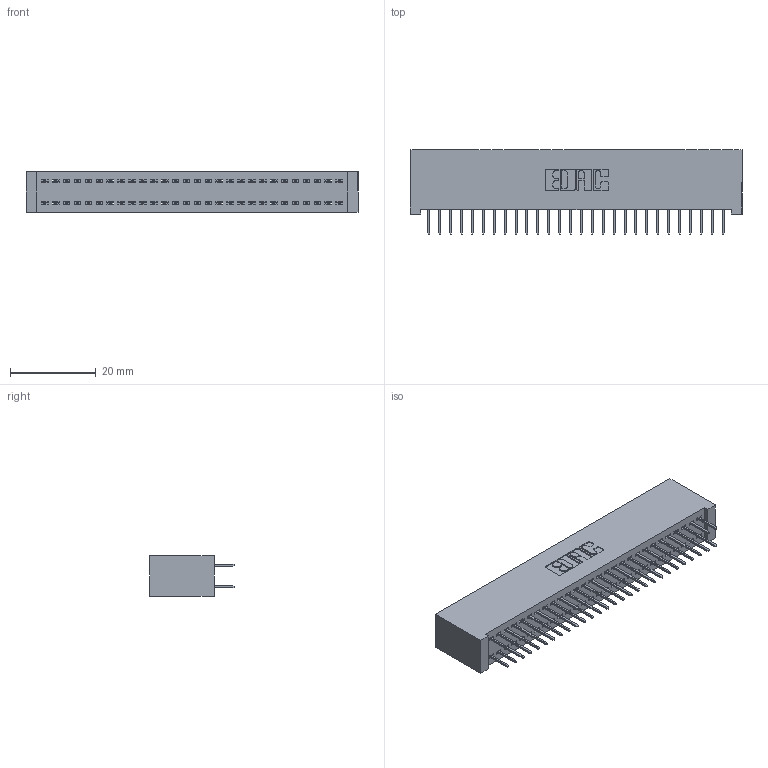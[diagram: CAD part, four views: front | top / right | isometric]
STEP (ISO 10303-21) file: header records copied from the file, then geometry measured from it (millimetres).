
FILE_DESCRIPTION (( 'STEP AP203' ), '1' );
FILE_NAME ('342-056-524-201.STEP', '2019-10-03T11:18:19', ( '' ), ( '' ), 'SwSTEP 2.0', 'SolidWorks 2016', '' );
FILE_SCHEMA (( 'CONFIG_CONTROL_DESIGN' ));
Length unit declared in the file: inch
Products named in the file (3): 342 Part_Lugless; 345-292-001_345-293-124; 342-056-524-201
Assembly tree (57 placements, depth 2):
  342-056-524-201
    342 Part_Lugless
    345-292-001_345-293-124  x56
Bounding box: 77.37 x 19.69 x 9.4 mm (x, y, z)
Volume: 7240 mm3; surface area: 11665.8 mm2
Topology: 57 solids, 57 shells, 3238 faces, 9179 edges, 5894 vertices
Faces by surface type: plane 2414, cylinder 824
Entity records: 19489 total; most frequent: CARTESIAN_POINT 3242, ORIENTED_EDGE 3178, DIRECTION 2789, EDGE_CURVE 1589, VECTOR 1473, LINE 1473, VERTEX_POINT 1054, AXIS2_PLACEMENT_3D 658
